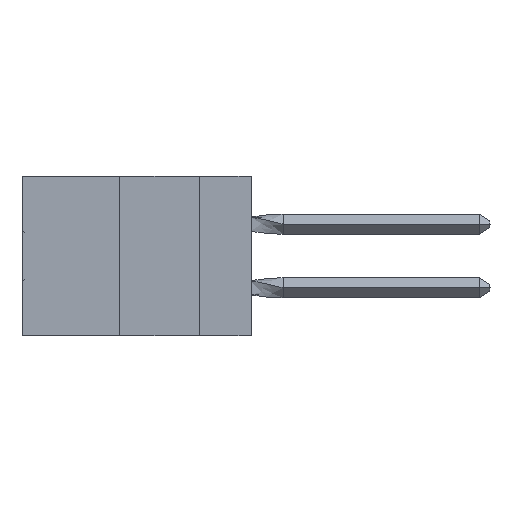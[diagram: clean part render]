
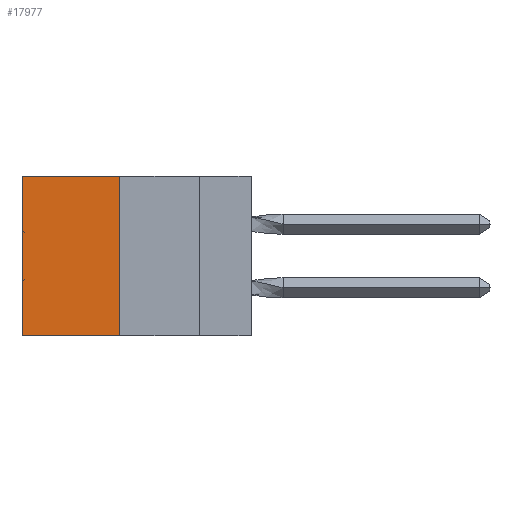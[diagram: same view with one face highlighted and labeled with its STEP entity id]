
A CAD part, left-side view. The second image highlights one B-rep face of the part: STEP entity #17977.
In plain terms, the highlighted planar face has unit normal (-1, 0, 0).
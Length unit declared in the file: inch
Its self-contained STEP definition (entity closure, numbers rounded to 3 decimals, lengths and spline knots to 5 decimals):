
#718 = DIRECTION ( 'NONE',  ( 1., 0., 0. ) ) ;
#1310 = LINE ( 'NONE', #2774, #1927 ) ;
#1771 = ORIENTED_EDGE ( 'NONE', *, *, #44971, .F. ) ;
#1927 = VECTOR ( 'NONE', #29088, 39.37008 ) ;
#2774 = CARTESIAN_POINT ( 'NONE',  ( 0.305, 0.72, -0.5 ) ) ;
#6174 = CARTESIAN_POINT ( 'NONE',  ( 0.305, 0.413, 0. ) ) ;
#7962 = DIRECTION ( 'NONE',  ( 0., 1., 0. ) ) ;
#9373 = AXIS2_PLACEMENT_3D ( 'NONE', #11895, #718, #26597 ) ;
#11091 = VERTEX_POINT ( 'NONE', #30722 ) ;
#11507 = FACE_OUTER_BOUND ( 'NONE', #15314, .T. ) ;
#11895 = CARTESIAN_POINT ( 'NONE',  ( 0.305, 0.413, -0.5 ) ) ;
#11983 = EDGE_CURVE ( 'NONE', #15847, #46560, #1310, .T. ) ;
#14398 = CARTESIAN_POINT ( 'NONE',  ( 0.305, 0.413, -0.5 ) ) ;
#15314 = EDGE_LOOP ( 'NONE', ( #23243, #1771, #18800, #36868 ) ) ;
#15847 = VERTEX_POINT ( 'NONE', #38910 ) ;
#16264 = LINE ( 'NONE', #23487, #36559 ) ;
#17977 = ADVANCED_FACE ( 'NONE', ( #11507 ), #38122, .F. ) ;
#18435 = VECTOR ( 'NONE', #29247, 39.37008 ) ;
#18494 = CARTESIAN_POINT ( 'NONE',  ( 0.305, 0.72, -0.5 ) ) ;
#18800 = ORIENTED_EDGE ( 'NONE', *, *, #46050, .F. ) ;
#19056 = CARTESIAN_POINT ( 'NONE',  ( 0.305, 0.413, 0. ) ) ;
#21284 = EDGE_CURVE ( 'NONE', #37900, #15847, #31726, .T. ) ;
#21822 = VECTOR ( 'NONE', #7962, 39.37008 ) ;
#23243 = ORIENTED_EDGE ( 'NONE', *, *, #11983, .T. ) ;
#23487 = CARTESIAN_POINT ( 'NONE',  ( 0.305, 0.413, -0.5 ) ) ;
#26597 = DIRECTION ( 'NONE',  ( 0., 0., -1. ) ) ;
#29088 = DIRECTION ( 'NONE',  ( 0., 0., -1. ) ) ;
#29247 = DIRECTION ( 'NONE',  ( 0., 0., -1. ) ) ;
#30282 = DIRECTION ( 'NONE',  ( 0., 1., 0. ) ) ;
#30722 = CARTESIAN_POINT ( 'NONE',  ( 0.305, 0.413, -0.5 ) ) ;
#31726 = LINE ( 'NONE', #19056, #21822 ) ;
#36559 = VECTOR ( 'NONE', #30282, 39.37008 ) ;
#36868 = ORIENTED_EDGE ( 'NONE', *, *, #21284, .T. ) ;
#37900 = VERTEX_POINT ( 'NONE', #6174 ) ;
#38122 = PLANE ( 'NONE',  #9373 ) ;
#38910 = CARTESIAN_POINT ( 'NONE',  ( 0.305, 0.72, 0. ) ) ;
#39373 = LINE ( 'NONE', #14398, #18435 ) ;
#44971 = EDGE_CURVE ( 'NONE', #11091, #46560, #16264, .T. ) ;
#46050 = EDGE_CURVE ( 'NONE', #37900, #11091, #39373, .T. ) ;
#46560 = VERTEX_POINT ( 'NONE', #18494 ) ;
